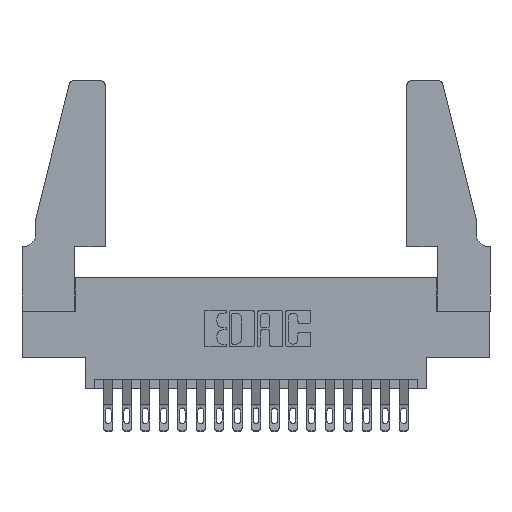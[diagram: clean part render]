
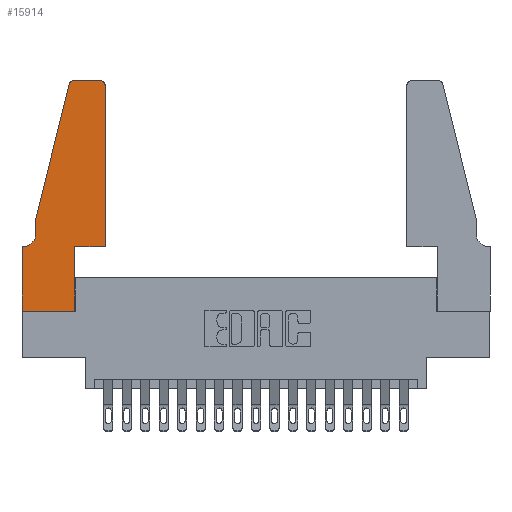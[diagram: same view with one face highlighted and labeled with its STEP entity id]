
A CAD part, top view. The second image highlights one B-rep face of the part: STEP entity #15914.
In plain terms, the highlighted planar face has unit normal (0, 0, 1).
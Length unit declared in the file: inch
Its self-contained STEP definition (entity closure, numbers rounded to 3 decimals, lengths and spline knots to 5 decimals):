
#102 = CARTESIAN_POINT ( 'NONE',  ( 0.2605, 1.25, 0.37 ) ) ;
#168 = CARTESIAN_POINT ( 'NONE',  ( 0.4205, 1.22, 0.37 ) ) ;
#303 = DIRECTION ( 'NONE',  ( 1., 0., 0. ) ) ;
#653 = DIRECTION ( 'NONE',  ( 1., 0., 0. ) ) ;
#784 = EDGE_CURVE ( 'NONE', #18782, #10272, #3035, .T. ) ;
#920 = DIRECTION ( 'NONE',  ( -0.239, -0.971, 0. ) ) ;
#960 = DIRECTION ( 'NONE',  ( 0., -1., 0. ) ) ;
#1052 = ORIENTED_EDGE ( 'NONE', *, *, #14990, .T. ) ;
#1138 = DIRECTION ( 'NONE',  ( -1., 0., 0. ) ) ;
#1158 = DIRECTION ( 'NONE',  ( 0., 0., -1. ) ) ;
#1176 = CARTESIAN_POINT ( 'NONE',  ( 0.0055, 0.42, 0.37 ) ) ;
#1235 = EDGE_CURVE ( 'NONE', #15466, #18964, #18296, .T. ) ;
#1595 = CARTESIAN_POINT ( 'NONE',  ( 0., 0., 0.37 ) ) ;
#1720 = DIRECTION ( 'NONE',  ( 1., 0., 0. ) ) ;
#1830 = EDGE_CURVE ( 'NONE', #6412, #8994, #13542, .T. ) ;
#1874 = ORIENTED_EDGE ( 'NONE', *, *, #6404, .T. ) ;
#2013 = EDGE_CURVE ( 'NONE', #18964, #4115, #10280, .T. ) ;
#2074 = DIRECTION ( 'NONE',  ( 1., 0., 0. ) ) ;
#2429 = CARTESIAN_POINT ( 'NONE',  ( 0.4505, 0.35, 0.37 ) ) ;
#2488 = VERTEX_POINT ( 'NONE', #3422 ) ;
#2693 = VERTEX_POINT ( 'NONE', #8471 ) ;
#2969 = ORIENTED_EDGE ( 'NONE', *, *, #3907, .T. ) ;
#3031 = VECTOR ( 'NONE', #15079, 39.37008 ) ;
#3035 = LINE ( 'NONE', #9736, #10560 ) ;
#3422 = CARTESIAN_POINT ( 'NONE',  ( 0., 0., 0.37 ) ) ;
#3907 = EDGE_CURVE ( 'NONE', #2488, #10501, #14376, .T. ) ;
#4115 = VERTEX_POINT ( 'NONE', #4153 ) ;
#4153 = CARTESIAN_POINT ( 'NONE',  ( 0.0755, 0.5, 0.37 ) ) ;
#4330 = CARTESIAN_POINT ( 'NONE',  ( 0., 0.35, 0.37 ) ) ;
#4358 = DIRECTION ( 'NONE',  ( -1., 0., 0. ) ) ;
#4486 = AXIS2_PLACEMENT_3D ( 'NONE', #1176, #1158, #1138 ) ;
#4643 = ORIENTED_EDGE ( 'NONE', *, *, #18088, .T. ) ;
#4776 = CARTESIAN_POINT ( 'NONE',  ( 0.2865, 0.35, 0.37 ) ) ;
#4802 = CARTESIAN_POINT ( 'NONE',  ( 0.4505, 0.35, 0.37 ) ) ;
#5846 = VECTOR ( 'NONE', #920, 39.37008 ) ;
#6119 = AXIS2_PLACEMENT_3D ( 'NONE', #4330, #7336, #17660 ) ;
#6253 = ORIENTED_EDGE ( 'NONE', *, *, #1235, .T. ) ;
#6404 = EDGE_CURVE ( 'NONE', #14258, #15466, #15416, .T. ) ;
#6412 = VERTEX_POINT ( 'NONE', #16533 ) ;
#6432 = VECTOR ( 'NONE', #4358, 39.37008 ) ;
#6490 = VECTOR ( 'NONE', #653, 39.37008 ) ;
#6699 = LINE ( 'NONE', #9133, #17995 ) ;
#6726 = CARTESIAN_POINT ( 'NONE',  ( 0., 0., 0.37 ) ) ;
#6728 = CARTESIAN_POINT ( 'NONE',  ( 0.25487, 1.22718, 0.37 ) ) ;
#6953 = EDGE_CURVE ( 'NONE', #10272, #9274, #13610, .T. ) ;
#7034 = LINE ( 'NONE', #1595, #3031 ) ;
#7336 = DIRECTION ( 'NONE',  ( 0., 0., 1. ) ) ;
#7591 = CARTESIAN_POINT ( 'NONE',  ( 0.4205, 1.25, 0.37 ) ) ;
#8017 = VECTOR ( 'NONE', #15081, 39.37008 ) ;
#8358 = ORIENTED_EDGE ( 'NONE', *, *, #1830, .T. ) ;
#8471 = CARTESIAN_POINT ( 'NONE',  ( 0., 0.35, 0.37 ) ) ;
#8503 = CARTESIAN_POINT ( 'NONE',  ( 0.0755, 0.5, 0.37 ) ) ;
#8583 = AXIS2_PLACEMENT_3D ( 'NONE', #168, #10794, #1720 ) ;
#8994 = VERTEX_POINT ( 'NONE', #18946 ) ;
#9131 = ORIENTED_EDGE ( 'NONE', *, *, #6953, .T. ) ;
#9133 = CARTESIAN_POINT ( 'NONE',  ( 0.2865, 0.35, 0.37 ) ) ;
#9274 = VERTEX_POINT ( 'NONE', #10700 ) ;
#9657 = VECTOR ( 'NONE', #10848, 39.37008 ) ;
#9736 = CARTESIAN_POINT ( 'NONE',  ( 0.4505, 0.35, 0.37 ) ) ;
#10272 = VERTEX_POINT ( 'NONE', #2429 ) ;
#10280 = LINE ( 'NONE', #8503, #5846 ) ;
#10492 = ORIENTED_EDGE ( 'NONE', *, *, #19202, .T. ) ;
#10501 = VERTEX_POINT ( 'NONE', #19292 ) ;
#10560 = VECTOR ( 'NONE', #2074, 39.37008 ) ;
#10700 = CARTESIAN_POINT ( 'NONE',  ( 0.4505, 1.22, 0.37 ) ) ;
#10794 = DIRECTION ( 'NONE',  ( 0., 0., 1. ) ) ;
#10839 = CARTESIAN_POINT ( 'NONE',  ( 0.284, 1.22, 0.37 ) ) ;
#10848 = DIRECTION ( 'NONE',  ( 0., 1., 0. ) ) ;
#11036 = CIRCLE ( 'NONE', #8583, 0.03 ) ;
#11478 = ORIENTED_EDGE ( 'NONE', *, *, #14934, .T. ) ;
#11877 = VECTOR ( 'NONE', #960, 39.37008 ) ;
#12597 = ORIENTED_EDGE ( 'NONE', *, *, #784, .T. ) ;
#13021 = EDGE_LOOP ( 'NONE', ( #1874, #6253, #16676, #13080, #8358, #10492, #11478, #2969, #4643, #12597, #9131, #1052 ) ) ;
#13080 = ORIENTED_EDGE ( 'NONE', *, *, #17798, .T. ) ;
#13264 = LINE ( 'NONE', #18816, #11877 ) ;
#13542 = CIRCLE ( 'NONE', #4486, 0.07 ) ;
#13610 = LINE ( 'NONE', #4802, #9657 ) ;
#13621 = DIRECTION ( 'NONE',  ( 0., 1., 0. ) ) ;
#13879 = LINE ( 'NONE', #17686, #6432 ) ;
#14258 = VERTEX_POINT ( 'NONE', #7591 ) ;
#14376 = LINE ( 'NONE', #6726, #6490 ) ;
#14934 = EDGE_CURVE ( 'NONE', #2693, #2488, #7034, .T. ) ;
#14990 = EDGE_CURVE ( 'NONE', #9274, #14258, #11036, .T. ) ;
#15079 = DIRECTION ( 'NONE',  ( 0., -1., 0. ) ) ;
#15081 = DIRECTION ( 'NONE',  ( -1., 0., 0. ) ) ;
#15416 = LINE ( 'NONE', #102, #8017 ) ;
#15466 = VERTEX_POINT ( 'NONE', #17926 ) ;
#15914 = ADVANCED_FACE ( 'NONE', ( #17842 ), #16178, .T. ) ;
#16138 = AXIS2_PLACEMENT_3D ( 'NONE', #10839, #16882, #303 ) ;
#16178 = PLANE ( 'NONE',  #6119 ) ;
#16533 = CARTESIAN_POINT ( 'NONE',  ( 0.0755, 0.42, 0.37 ) ) ;
#16676 = ORIENTED_EDGE ( 'NONE', *, *, #2013, .T. ) ;
#16882 = DIRECTION ( 'NONE',  ( 0., 0., 1. ) ) ;
#17660 = DIRECTION ( 'NONE',  ( 1., 0., 0. ) ) ;
#17686 = CARTESIAN_POINT ( 'NONE',  ( 0.0755, 0.35, 0.37 ) ) ;
#17798 = EDGE_CURVE ( 'NONE', #4115, #6412, #13264, .T. ) ;
#17842 = FACE_OUTER_BOUND ( 'NONE', #13021, .T. ) ;
#17926 = CARTESIAN_POINT ( 'NONE',  ( 0.284, 1.25, 0.37 ) ) ;
#17995 = VECTOR ( 'NONE', #13621, 39.37008 ) ;
#18088 = EDGE_CURVE ( 'NONE', #10501, #18782, #6699, .T. ) ;
#18296 = CIRCLE ( 'NONE', #16138, 0.03 ) ;
#18782 = VERTEX_POINT ( 'NONE', #4776 ) ;
#18816 = CARTESIAN_POINT ( 'NONE',  ( 0.0755, 0.5, 0.37 ) ) ;
#18946 = CARTESIAN_POINT ( 'NONE',  ( 0.0055, 0.35, 0.37 ) ) ;
#18964 = VERTEX_POINT ( 'NONE', #6728 ) ;
#19202 = EDGE_CURVE ( 'NONE', #8994, #2693, #13879, .T. ) ;
#19292 = CARTESIAN_POINT ( 'NONE',  ( 0.2865, 0., 0.37 ) ) ;
